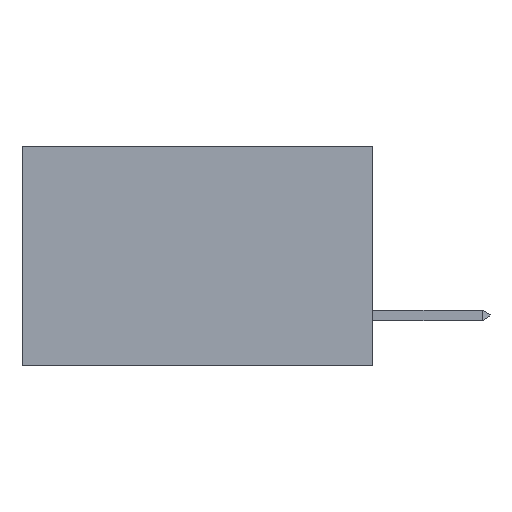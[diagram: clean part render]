
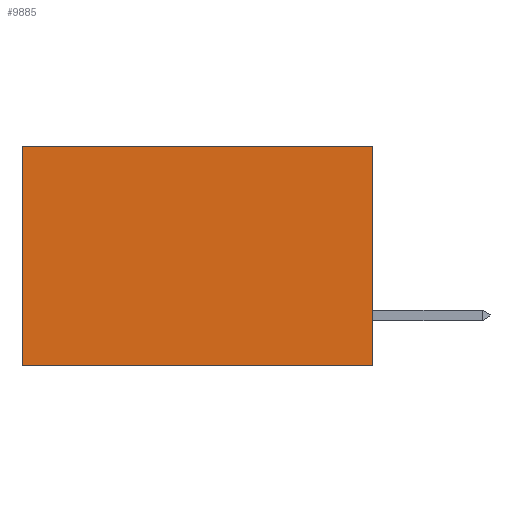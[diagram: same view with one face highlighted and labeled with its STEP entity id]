
A CAD part, left-side view. The second image highlights one B-rep face of the part: STEP entity #9885.
In plain terms, the highlighted planar face has unit normal (-1, 0, 0).
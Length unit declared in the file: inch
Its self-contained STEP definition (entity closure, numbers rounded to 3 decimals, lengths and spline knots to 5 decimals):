
#85 = VECTOR ( 'NONE', #1710, 39.37008 ) ;
#159 = PLANE ( 'NONE',  #6810 ) ;
#206 = DIRECTION ( 'NONE',  ( 1., 0., 0. ) ) ;
#291 = CARTESIAN_POINT ( 'NONE',  ( 0.277, 0., 0. ) ) ;
#1285 = LINE ( 'NONE', #3216, #6761 ) ;
#1529 = CARTESIAN_POINT ( 'NONE',  ( 0.277, 0., -0.37 ) ) ;
#1710 = DIRECTION ( 'NONE',  ( 0., 1., 0. ) ) ;
#2159 = EDGE_CURVE ( 'NONE', #10419, #11938, #7663, .T. ) ;
#2732 = ORIENTED_EDGE ( 'NONE', *, *, #2159, .T. ) ;
#3200 = DIRECTION ( 'NONE',  ( 0., 0., -1. ) ) ;
#3216 = CARTESIAN_POINT ( 'NONE',  ( 0.277, 0., -0.37 ) ) ;
#3655 = CARTESIAN_POINT ( 'NONE',  ( 0.277, 0.59, -0.37 ) ) ;
#3802 = DIRECTION ( 'NONE',  ( 0., 0., -1. ) ) ;
#4624 = VECTOR ( 'NONE', #11219, 39.37008 ) ;
#5114 = CARTESIAN_POINT ( 'NONE',  ( 0.277, 0., 0. ) ) ;
#5308 = CARTESIAN_POINT ( 'NONE',  ( 0.277, 0., -0.37 ) ) ;
#5929 = CARTESIAN_POINT ( 'NONE',  ( 0.277, 0.59, -0.37 ) ) ;
#6421 = EDGE_CURVE ( 'NONE', #10419, #11279, #1285, .T. ) ;
#6761 = VECTOR ( 'NONE', #3200, 39.37008 ) ;
#6810 = AXIS2_PLACEMENT_3D ( 'NONE', #5308, #206, #7368 ) ;
#7143 = LINE ( 'NONE', #3655, #9450 ) ;
#7368 = DIRECTION ( 'NONE',  ( 0., 0., -1. ) ) ;
#7663 = LINE ( 'NONE', #291, #4624 ) ;
#7835 = ORIENTED_EDGE ( 'NONE', *, *, #8423, .F. ) ;
#8143 = VERTEX_POINT ( 'NONE', #5929 ) ;
#8306 = EDGE_CURVE ( 'NONE', #11938, #8143, #7143, .T. ) ;
#8423 = EDGE_CURVE ( 'NONE', #11279, #8143, #10767, .T. ) ;
#9450 = VECTOR ( 'NONE', #3802, 39.37008 ) ;
#9653 = EDGE_LOOP ( 'NONE', ( #12614, #7835, #10397, #2732 ) ) ;
#9885 = ADVANCED_FACE ( 'NONE', ( #12058 ), #159, .F. ) ;
#10397 = ORIENTED_EDGE ( 'NONE', *, *, #6421, .F. ) ;
#10419 = VERTEX_POINT ( 'NONE', #5114 ) ;
#10767 = LINE ( 'NONE', #1529, #85 ) ;
#11219 = DIRECTION ( 'NONE',  ( 0., 1., 0. ) ) ;
#11279 = VERTEX_POINT ( 'NONE', #11332 ) ;
#11332 = CARTESIAN_POINT ( 'NONE',  ( 0.277, 0., -0.37 ) ) ;
#11938 = VERTEX_POINT ( 'NONE', #12522 ) ;
#12058 = FACE_OUTER_BOUND ( 'NONE', #9653, .T. ) ;
#12522 = CARTESIAN_POINT ( 'NONE',  ( 0.277, 0.59, 0. ) ) ;
#12614 = ORIENTED_EDGE ( 'NONE', *, *, #8306, .T. ) ;
